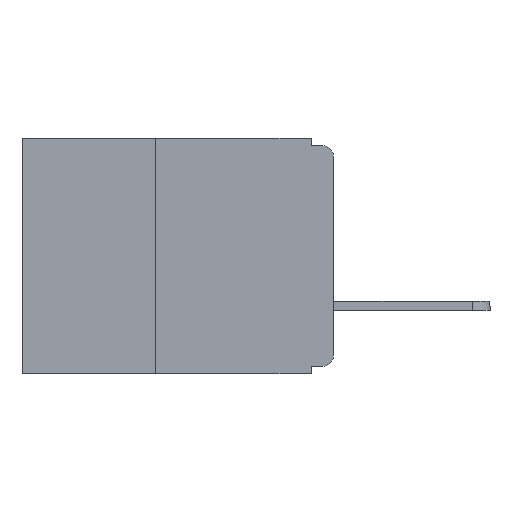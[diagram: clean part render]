
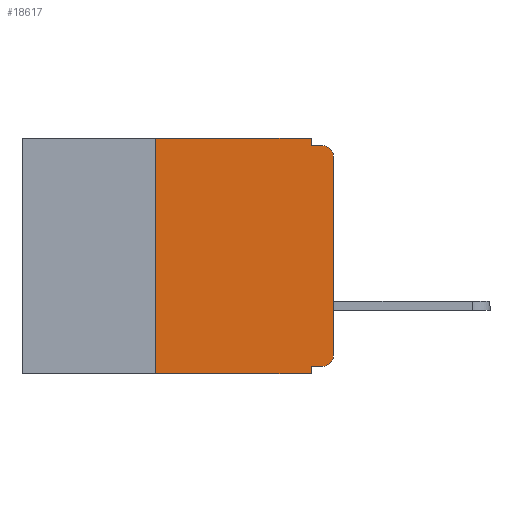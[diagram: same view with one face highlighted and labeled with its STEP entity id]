
A CAD part, left-side view. The second image highlights one B-rep face of the part: STEP entity #18617.
In plain terms, the highlighted planar face has unit normal (-1, 0, 0).
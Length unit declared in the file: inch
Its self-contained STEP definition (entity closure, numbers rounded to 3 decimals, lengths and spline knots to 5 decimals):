
#189 = VECTOR ( 'NONE', #3986, 39.37008 ) ;
#473 = VECTOR ( 'NONE', #18815, 39.37008 ) ;
#737 = LINE ( 'NONE', #21089, #189 ) ;
#1260 = CARTESIAN_POINT ( 'NONE',  ( 0., 0.031, 0. ) ) ;
#2189 = ORIENTED_EDGE ( 'NONE', *, *, #10580, .F. ) ;
#2628 = EDGE_CURVE ( 'NONE', #4389, #11721, #6523, .T. ) ;
#2752 = CARTESIAN_POINT ( 'NONE',  ( 0., 0., 0. ) ) ;
#2891 = VERTEX_POINT ( 'NONE', #11203 ) ;
#2910 = VECTOR ( 'NONE', #15129, 39.37008 ) ;
#3004 = CARTESIAN_POINT ( 'NONE',  ( 0., 0.031, 0. ) ) ;
#3074 = EDGE_CURVE ( 'NONE', #5423, #5294, #10518, .T. ) ;
#3319 = ORIENTED_EDGE ( 'NONE', *, *, #13350, .T. ) ;
#3986 = DIRECTION ( 'NONE',  ( 0., 0., -1. ) ) ;
#4290 = VECTOR ( 'NONE', #7415, 39.37008 ) ;
#4328 = EDGE_CURVE ( 'NONE', #4901, #5423, #6974, .T. ) ;
#4351 = LINE ( 'NONE', #12319, #12446 ) ;
#4389 = VERTEX_POINT ( 'NONE', #9036 ) ;
#4508 = DIRECTION ( 'NONE',  ( 0., 0., 1. ) ) ;
#4901 = VERTEX_POINT ( 'NONE', #21143 ) ;
#5294 = VERTEX_POINT ( 'NONE', #6975 ) ;
#5423 = VERTEX_POINT ( 'NONE', #1260 ) ;
#5429 = VECTOR ( 'NONE', #11577, 39.37008 ) ;
#5481 = ORIENTED_EDGE ( 'NONE', *, *, #12906, .F. ) ;
#5747 = ORIENTED_EDGE ( 'NONE', *, *, #22083, .T. ) ;
#5947 = CARTESIAN_POINT ( 'NONE',  ( 0., 0.015, -0.025 ) ) ;
#6324 = CARTESIAN_POINT ( 'NONE',  ( 0., 0.031, -0.32 ) ) ;
#6523 = LINE ( 'NONE', #2752, #10545 ) ;
#6563 = CARTESIAN_POINT ( 'NONE',  ( 0., 0.015, -0.32 ) ) ;
#6974 = LINE ( 'NONE', #19052, #2910 ) ;
#6975 = CARTESIAN_POINT ( 'NONE',  ( 0., 0.031, -0.01 ) ) ;
#7415 = DIRECTION ( 'NONE',  ( 0., -1., 0. ) ) ;
#7651 = VERTEX_POINT ( 'NONE', #11236 ) ;
#7677 = DIRECTION ( 'NONE',  ( 0., 0., -1. ) ) ;
#8164 = CARTESIAN_POINT ( 'NONE',  ( 0., 0.437, 0. ) ) ;
#8432 = ORIENTED_EDGE ( 'NONE', *, *, #3074, .F. ) ;
#8459 = EDGE_CURVE ( 'NONE', #7651, #2891, #8904, .T. ) ;
#8882 = VERTEX_POINT ( 'NONE', #11918 ) ;
#8904 = LINE ( 'NONE', #19371, #4290 ) ;
#9036 = CARTESIAN_POINT ( 'NONE',  ( 0., 0., -0.305 ) ) ;
#9252 = ORIENTED_EDGE ( 'NONE', *, *, #13108, .F. ) ;
#9780 = DIRECTION ( 'NONE',  ( -1., 0., 0. ) ) ;
#9869 = DIRECTION ( 'NONE',  ( 0., 0., -1. ) ) ;
#10385 = FACE_OUTER_BOUND ( 'NONE', #15098, .T. ) ;
#10518 = LINE ( 'NONE', #3004, #5429 ) ;
#10545 = VECTOR ( 'NONE', #4508, 39.37008 ) ;
#10580 = EDGE_CURVE ( 'NONE', #5294, #8882, #13648, .T. ) ;
#11203 = CARTESIAN_POINT ( 'NONE',  ( 0., 0.031, -0.33 ) ) ;
#11236 = CARTESIAN_POINT ( 'NONE',  ( 0., 0.25, -0.33 ) ) ;
#11551 = VERTEX_POINT ( 'NONE', #6324 ) ;
#11577 = DIRECTION ( 'NONE',  ( 0., 0., -1. ) ) ;
#11721 = VERTEX_POINT ( 'NONE', #17305 ) ;
#11918 = CARTESIAN_POINT ( 'NONE',  ( 0., 0.015, -0.01 ) ) ;
#12191 = ORIENTED_EDGE ( 'NONE', *, *, #2628, .T. ) ;
#12319 = CARTESIAN_POINT ( 'NONE',  ( 0., 0., -0.32 ) ) ;
#12446 = VECTOR ( 'NONE', #14009, 39.37008 ) ;
#12906 = EDGE_CURVE ( 'NONE', #7651, #4901, #13799, .T. ) ;
#13108 = EDGE_CURVE ( 'NONE', #11551, #2891, #737, .T. ) ;
#13350 = EDGE_CURVE ( 'NONE', #21692, #4389, #22250, .T. ) ;
#13648 = LINE ( 'NONE', #21549, #18160 ) ;
#13799 = LINE ( 'NONE', #15381, #473 ) ;
#14009 = DIRECTION ( 'NONE',  ( 0., 1., 0. ) ) ;
#14234 = AXIS2_PLACEMENT_3D ( 'NONE', #8164, #20077, #9869 ) ;
#15098 = EDGE_LOOP ( 'NONE', ( #12191, #5747, #2189, #8432, #18040, #5481, #17259, #9252, #15945, #3319 ) ) ;
#15129 = DIRECTION ( 'NONE',  ( 0., -1., 0. ) ) ;
#15241 = EDGE_CURVE ( 'NONE', #21692, #11551, #4351, .T. ) ;
#15381 = CARTESIAN_POINT ( 'NONE',  ( 0., 0.25, -0.33 ) ) ;
#15569 = AXIS2_PLACEMENT_3D ( 'NONE', #5947, #17889, #7677 ) ;
#15945 = ORIENTED_EDGE ( 'NONE', *, *, #15241, .F. ) ;
#17259 = ORIENTED_EDGE ( 'NONE', *, *, #8459, .T. ) ;
#17305 = CARTESIAN_POINT ( 'NONE',  ( 0., 0., -0.025 ) ) ;
#17774 = AXIS2_PLACEMENT_3D ( 'NONE', #19984, #9780, #21662 ) ;
#17889 = DIRECTION ( 'NONE',  ( -1., 0., 0. ) ) ;
#18040 = ORIENTED_EDGE ( 'NONE', *, *, #4328, .F. ) ;
#18158 = DIRECTION ( 'NONE',  ( 0., -1., 0. ) ) ;
#18160 = VECTOR ( 'NONE', #18158, 39.37008 ) ;
#18372 = PLANE ( 'NONE',  #14234 ) ;
#18617 = ADVANCED_FACE ( 'NONE', ( #10385 ), #18372, .F. ) ;
#18782 = CIRCLE ( 'NONE', #15569, 0.015 ) ;
#18815 = DIRECTION ( 'NONE',  ( 0., 0., 1. ) ) ;
#19052 = CARTESIAN_POINT ( 'NONE',  ( 0., 0.437, 0. ) ) ;
#19371 = CARTESIAN_POINT ( 'NONE',  ( 0., 0.437, -0.33 ) ) ;
#19984 = CARTESIAN_POINT ( 'NONE',  ( 0., 0.015, -0.305 ) ) ;
#20077 = DIRECTION ( 'NONE',  ( 1., 0., 0. ) ) ;
#21089 = CARTESIAN_POINT ( 'NONE',  ( 0., 0.031, -0.33 ) ) ;
#21143 = CARTESIAN_POINT ( 'NONE',  ( 0., 0.25, 0. ) ) ;
#21549 = CARTESIAN_POINT ( 'NONE',  ( 0., 0., -0.01 ) ) ;
#21662 = DIRECTION ( 'NONE',  ( 0., 0., -1. ) ) ;
#21692 = VERTEX_POINT ( 'NONE', #6563 ) ;
#22083 = EDGE_CURVE ( 'NONE', #11721, #8882, #18782, .T. ) ;
#22250 = CIRCLE ( 'NONE', #17774, 0.015 ) ;
